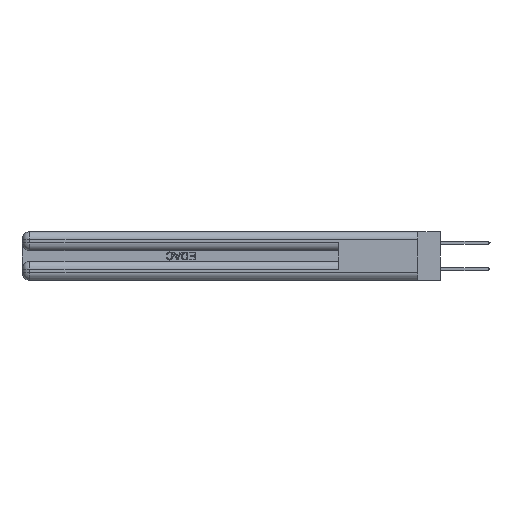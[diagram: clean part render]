
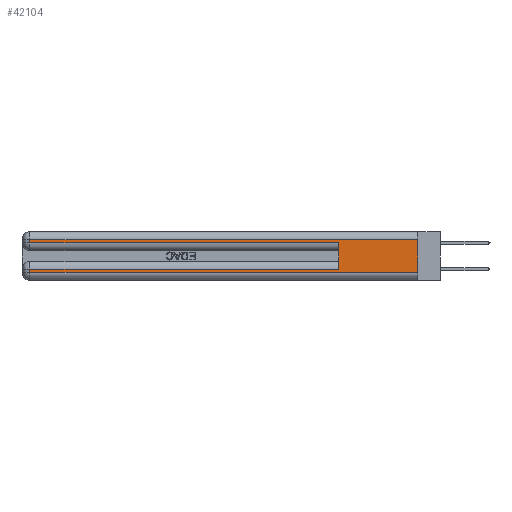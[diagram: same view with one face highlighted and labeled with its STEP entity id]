
A CAD part, left-side view. The second image highlights one B-rep face of the part: STEP entity #42104.
In plain terms, the highlighted planar face has unit normal (-1, 0, 0).
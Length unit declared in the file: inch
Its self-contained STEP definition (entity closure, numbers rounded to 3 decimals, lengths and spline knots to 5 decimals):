
#710 = VERTEX_POINT ( 'NONE', #2199 ) ;
#1508 = VECTOR ( 'NONE', #18927, 39.37008 ) ;
#1530 = ORIENTED_EDGE ( 'NONE', *, *, #5385, .T. ) ;
#1602 = DIRECTION ( 'NONE',  ( 0., 0., 1. ) ) ;
#1706 = EDGE_CURVE ( 'NONE', #37683, #45335, #27716, .T. ) ;
#2199 = CARTESIAN_POINT ( 'NONE',  ( 0., 2.94, 0.06 ) ) ;
#2909 = CARTESIAN_POINT ( 'NONE',  ( 0., 0.6, 0.085 ) ) ;
#3057 = VERTEX_POINT ( 'NONE', #2909 ) ;
#4294 = EDGE_CURVE ( 'NONE', #3057, #7005, #6835, .T. ) ;
#5243 = LINE ( 'NONE', #13850, #27499 ) ;
#5385 = EDGE_CURVE ( 'NONE', #37683, #24186, #30813, .T. ) ;
#6412 = CARTESIAN_POINT ( 'NONE',  ( 0., 0.6, 0.285 ) ) ;
#6835 = LINE ( 'NONE', #29255, #27855 ) ;
#7005 = VERTEX_POINT ( 'NONE', #6412 ) ;
#8779 = EDGE_CURVE ( 'NONE', #28339, #710, #31796, .T. ) ;
#13343 = LINE ( 'NONE', #22719, #1508 ) ;
#13850 = CARTESIAN_POINT ( 'NONE',  ( 0., 0., 0.085 ) ) ;
#15129 = ORIENTED_EDGE ( 'NONE', *, *, #33620, .T. ) ;
#15387 = PLANE ( 'NONE',  #31351 ) ;
#16600 = ORIENTED_EDGE ( 'NONE', *, *, #1706, .F. ) ;
#18927 = DIRECTION ( 'NONE',  ( 0., 0., -1. ) ) ;
#18973 = DIRECTION ( 'NONE',  ( 0., -1., 0. ) ) ;
#20286 = ORIENTED_EDGE ( 'NONE', *, *, #4294, .F. ) ;
#20578 = DIRECTION ( 'NONE',  ( 0., 1., 0. ) ) ;
#21322 = VECTOR ( 'NONE', #38893, 39.37008 ) ;
#21870 = ORIENTED_EDGE ( 'NONE', *, *, #23253, .T. ) ;
#21928 = DIRECTION ( 'NONE',  ( 0., 1., 0. ) ) ;
#22719 = CARTESIAN_POINT ( 'NONE',  ( 0., 2.94, 0.37 ) ) ;
#23012 = CARTESIAN_POINT ( 'NONE',  ( 0., 2.94, 0.37 ) ) ;
#23253 = EDGE_CURVE ( 'NONE', #24186, #27452, #13343, .T. ) ;
#23291 = DIRECTION ( 'NONE',  ( 1., 0., 0. ) ) ;
#24186 = VERTEX_POINT ( 'NONE', #28969 ) ;
#26810 = EDGE_LOOP ( 'NONE', ( #16600, #1530, #21870, #40024, #20286, #47255, #38591, #15129 ) ) ;
#27452 = VERTEX_POINT ( 'NONE', #45389 ) ;
#27499 = VECTOR ( 'NONE', #21928, 39.37008 ) ;
#27716 = LINE ( 'NONE', #34500, #47555 ) ;
#27855 = VECTOR ( 'NONE', #1602, 39.37008 ) ;
#28339 = VERTEX_POINT ( 'NONE', #51189 ) ;
#28969 = CARTESIAN_POINT ( 'NONE',  ( 0., 2.94, 0.31 ) ) ;
#29255 = CARTESIAN_POINT ( 'NONE',  ( 0., 0.6, 0.145 ) ) ;
#30813 = LINE ( 'NONE', #40261, #50692 ) ;
#31351 = AXIS2_PLACEMENT_3D ( 'NONE', #47007, #23291, #50998 ) ;
#31796 = LINE ( 'NONE', #23012, #21322 ) ;
#33620 = EDGE_CURVE ( 'NONE', #710, #45335, #47692, .T. ) ;
#34500 = CARTESIAN_POINT ( 'NONE',  ( 0., 0., 0.37 ) ) ;
#34675 = CARTESIAN_POINT ( 'NONE',  ( 0., 0., 0.06 ) ) ;
#36136 = VECTOR ( 'NONE', #36374, 39.37008 ) ;
#36374 = DIRECTION ( 'NONE',  ( 0., -1., 0. ) ) ;
#37683 = VERTEX_POINT ( 'NONE', #46995 ) ;
#38591 = ORIENTED_EDGE ( 'NONE', *, *, #8779, .T. ) ;
#38893 = DIRECTION ( 'NONE',  ( 0., 0., -1. ) ) ;
#40024 = ORIENTED_EDGE ( 'NONE', *, *, #49423, .T. ) ;
#40261 = CARTESIAN_POINT ( 'NONE',  ( 0., 0., 0.31 ) ) ;
#42104 = ADVANCED_FACE ( 'NONE', ( #45230 ), #15387, .F. ) ;
#42471 = DIRECTION ( 'NONE',  ( 0., 0., -1. ) ) ;
#42931 = CARTESIAN_POINT ( 'NONE',  ( 0., 0., 0.06 ) ) ;
#45230 = FACE_OUTER_BOUND ( 'NONE', #26810, .T. ) ;
#45335 = VERTEX_POINT ( 'NONE', #42931 ) ;
#45389 = CARTESIAN_POINT ( 'NONE',  ( 0., 2.94, 0.285 ) ) ;
#46386 = EDGE_CURVE ( 'NONE', #3057, #28339, #5243, .T. ) ;
#46452 = VECTOR ( 'NONE', #18973, 39.37008 ) ;
#46995 = CARTESIAN_POINT ( 'NONE',  ( 0., 0., 0.31 ) ) ;
#47007 = CARTESIAN_POINT ( 'NONE',  ( 0., 0., 0.37 ) ) ;
#47255 = ORIENTED_EDGE ( 'NONE', *, *, #46386, .T. ) ;
#47555 = VECTOR ( 'NONE', #42471, 39.37008 ) ;
#47692 = LINE ( 'NONE', #34675, #46452 ) ;
#47929 = LINE ( 'NONE', #48168, #36136 ) ;
#48168 = CARTESIAN_POINT ( 'NONE',  ( 0., 0., 0.285 ) ) ;
#49423 = EDGE_CURVE ( 'NONE', #27452, #7005, #47929, .T. ) ;
#50692 = VECTOR ( 'NONE', #20578, 39.37008 ) ;
#50998 = DIRECTION ( 'NONE',  ( 0., 0., -1. ) ) ;
#51189 = CARTESIAN_POINT ( 'NONE',  ( 0., 2.94, 0.085 ) ) ;
